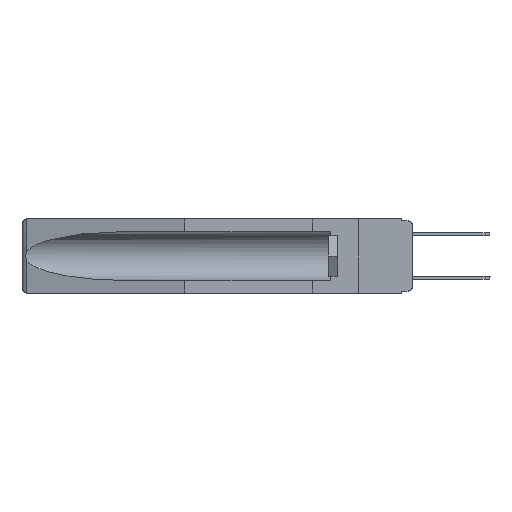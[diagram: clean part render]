
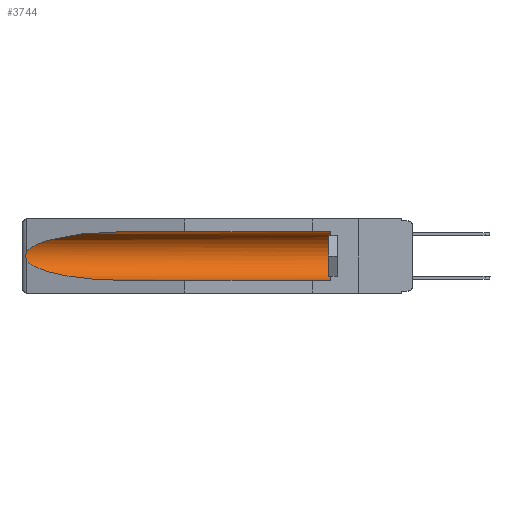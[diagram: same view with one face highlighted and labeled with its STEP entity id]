
A CAD part, left-side view. The second image highlights one B-rep face of the part: STEP entity #3744.
In plain terms, the highlighted cylindrical face has radius 2.857 mm (diameter 5.715 mm), a partial arc.
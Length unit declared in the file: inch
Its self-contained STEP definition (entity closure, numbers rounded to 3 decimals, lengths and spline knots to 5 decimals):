
#129 = CARTESIAN_POINT ( 'NONE',  ( 0.155, -0.30754, -0.059 ) ) ;
#562 = B_SPLINE_CURVE_WITH_KNOTS ( 'NONE', 3,
 ( #6955, #14461, #2624, #2563, #3973, #3914, #7082, #11543, #17408, #2684 ),
 .UNSPECIFIED., .F., .F.,
 ( 4, 2, 2, 2, 4 ),
 ( 0., 0.00029, 0.00058, 0.00087, 0.00117 ),
 .UNSPECIFIED. ) ;
#972 = AXIS2_PLACEMENT_3D ( 'NONE', #5123, #17000, #5187 ) ;
#1264 = CARTESIAN_POINT ( 'NONE',  ( 0.155, -0.30754, -0.284 ) ) ;
#1671 = ORIENTED_EDGE ( 'NONE', *, *, #18969, .F. ) ;
#1677 = CARTESIAN_POINT ( 'NONE',  ( 0.155, 1.07973, -0.059 ) ) ;
#2268 = VECTOR ( 'NONE', #13168, 39.37008 ) ;
#2563 = CARTESIAN_POINT ( 'NONE',  ( 0.2673, 1.5327, -0.16383 ) ) ;
#2624 = CARTESIAN_POINT ( 'NONE',  ( 0.26654, 1.53092, -0.15636 ) ) ;
#2684 = CARTESIAN_POINT ( 'NONE',  ( 0.26537, 1.52718, -0.19328 ) ) ;
#2753 = ORIENTED_EDGE ( 'NONE', *, *, #11441, .T. ) ;
#2785 = ORIENTED_EDGE ( 'NONE', *, *, #15042, .T. ) ;
#3223 = CARTESIAN_POINT ( 'NONE',  ( 0.155, 0.126, -0.1715 ) ) ;
#3744 = ADVANCED_FACE ( 'NONE', ( #15411 ), #7540, .F. ) ;
#3914 = CARTESIAN_POINT ( 'NONE',  ( 0.2675, 1.53308, -0.17534 ) ) ;
#3973 = CARTESIAN_POINT ( 'NONE',  ( 0.2675, 1.53308, -0.16763 ) ) ;
#4917 = CARTESIAN_POINT ( 'NONE',  ( 0.21114, 1.30732, -0.284 ) ) ;
#4980 = CARTESIAN_POINT ( 'NONE',  ( 0.155, 1.07973, -0.284 ) ) ;
#5123 = CARTESIAN_POINT ( 'NONE',  ( 0.155, -0.30754, -0.1715 ) ) ;
#5187 = DIRECTION ( 'NONE',  ( 0., 0., 1. ) ) ;
#5572 = VERTEX_POINT ( 'NONE', #12680 ) ;
#5765 =( BOUNDED_CURVE ( )  B_SPLINE_CURVE ( 3, ( #9196, #6088, #10675, #7682 ),
 .UNSPECIFIED., .F., .F. ) 
 B_SPLINE_CURVE_WITH_KNOTS ( ( 4, 4 ),
 ( 4.71239, 6.08839 ),
 .UNSPECIFIED. ) 
 CURVE ( )  GEOMETRIC_REPRESENTATION_ITEM ( )  RATIONAL_B_SPLINE_CURVE ( ( 1., 0.848, 0.848, 1. ) ) 
 REPRESENTATION_ITEM ( '' )  );
#5778 = CIRCLE ( 'NONE', #12158, 0.1125 ) ;
#6088 = CARTESIAN_POINT ( 'NONE',  ( 0.21114, 1.30732, -0.059 ) ) ;
#6955 = CARTESIAN_POINT ( 'NONE',  ( 0.26537, 1.52718, -0.14972 ) ) ;
#7082 = CARTESIAN_POINT ( 'NONE',  ( 0.2673, 1.53269, -0.17917 ) ) ;
#7441 = LINE ( 'NONE', #129, #8839 ) ;
#7540 = CYLINDRICAL_SURFACE ( 'NONE', #972, 0.1125 ) ;
#7682 = CARTESIAN_POINT ( 'NONE',  ( 0.26537, 1.52718, -0.14972 ) ) ;
#8839 = VECTOR ( 'NONE', #17866, 39.37008 ) ;
#8963 = EDGE_CURVE ( 'NONE', #5572, #17399, #7441, .T. ) ;
#9196 = CARTESIAN_POINT ( 'NONE',  ( 0.155, 1.07973, -0.059 ) ) ;
#9257 = DIRECTION ( 'NONE',  ( 0., 0., 1. ) ) ;
#9267 = CARTESIAN_POINT ( 'NONE',  ( 0.26537, 1.52718, -0.19328 ) ) ;
#9755 = CARTESIAN_POINT ( 'NONE',  ( 0.155, 1.07973, -0.284 ) ) ;
#9893 = LINE ( 'NONE', #1264, #2268 ) ;
#10484 = ORIENTED_EDGE ( 'NONE', *, *, #15994, .T. ) ;
#10675 = CARTESIAN_POINT ( 'NONE',  ( 0.25451, 1.48313, -0.09465 ) ) ;
#11441 = EDGE_CURVE ( 'NONE', #17399, #13195, #5765, .T. ) ;
#11543 = CARTESIAN_POINT ( 'NONE',  ( 0.26655, 1.53094, -0.18657 ) ) ;
#12158 = AXIS2_PLACEMENT_3D ( 'NONE', #3223, #13644, #9257 ) ;
#12591 = CARTESIAN_POINT ( 'NONE',  ( 0.26537, 1.52718, -0.19328 ) ) ;
#12680 = CARTESIAN_POINT ( 'NONE',  ( 0.155, 0.126, -0.059 ) ) ;
#12940 = CARTESIAN_POINT ( 'NONE',  ( 0.155, 0.126, -0.284 ) ) ;
#13168 = DIRECTION ( 'NONE',  ( 0., 1., 0. ) ) ;
#13195 = VERTEX_POINT ( 'NONE', #14321 ) ;
#13644 = DIRECTION ( 'NONE',  ( 0., -1., 0. ) ) ;
#13914 = VERTEX_POINT ( 'NONE', #12940 ) ;
#14321 = CARTESIAN_POINT ( 'NONE',  ( 0.26537, 1.52718, -0.14972 ) ) ;
#14461 = CARTESIAN_POINT ( 'NONE',  ( 0.26597, 1.52961, -0.15275 ) ) ;
#15042 = EDGE_CURVE ( 'NONE', #15837, #18303, #15474, .T. ) ;
#15075 = CARTESIAN_POINT ( 'NONE',  ( 0.25451, 1.48313, -0.24835 ) ) ;
#15411 = FACE_OUTER_BOUND ( 'NONE', #16575, .T. ) ;
#15474 =( BOUNDED_CURVE ( )  B_SPLINE_CURVE ( 3, ( #9267, #15075, #4917, #4980 ),
 .UNSPECIFIED., .F., .F. ) 
 B_SPLINE_CURVE_WITH_KNOTS ( ( 4, 4 ),
 ( 0.1948, 1.5708 ),
 .UNSPECIFIED. ) 
 CURVE ( )  GEOMETRIC_REPRESENTATION_ITEM ( )  RATIONAL_B_SPLINE_CURVE ( ( 1., 0.848, 0.848, 1. ) ) 
 REPRESENTATION_ITEM ( '' )  );
#15837 = VERTEX_POINT ( 'NONE', #12591 ) ;
#15994 = EDGE_CURVE ( 'NONE', #13195, #15837, #562, .T. ) ;
#16575 = EDGE_LOOP ( 'NONE', ( #2753, #10484, #2785, #1671, #16643, #17860 ) ) ;
#16643 = ORIENTED_EDGE ( 'NONE', *, *, #18022, .T. ) ;
#17000 = DIRECTION ( 'NONE',  ( 0., 1., 0. ) ) ;
#17399 = VERTEX_POINT ( 'NONE', #1677 ) ;
#17408 = CARTESIAN_POINT ( 'NONE',  ( 0.26597, 1.5296, -0.19026 ) ) ;
#17860 = ORIENTED_EDGE ( 'NONE', *, *, #8963, .T. ) ;
#17866 = DIRECTION ( 'NONE',  ( 0., 1., 0. ) ) ;
#18022 = EDGE_CURVE ( 'NONE', #13914, #5572, #5778, .T. ) ;
#18303 = VERTEX_POINT ( 'NONE', #9755 ) ;
#18969 = EDGE_CURVE ( 'NONE', #13914, #18303, #9893, .T. ) ;
